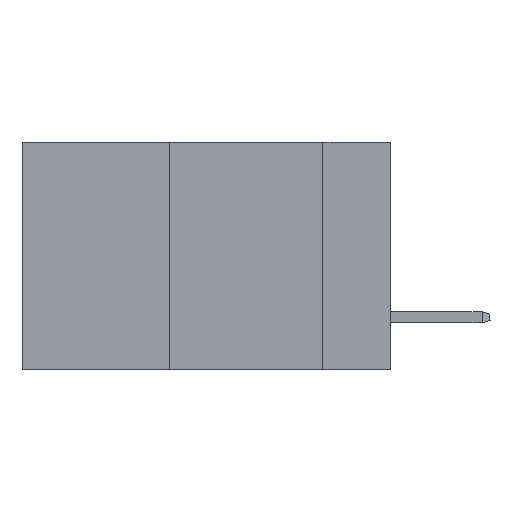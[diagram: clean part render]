
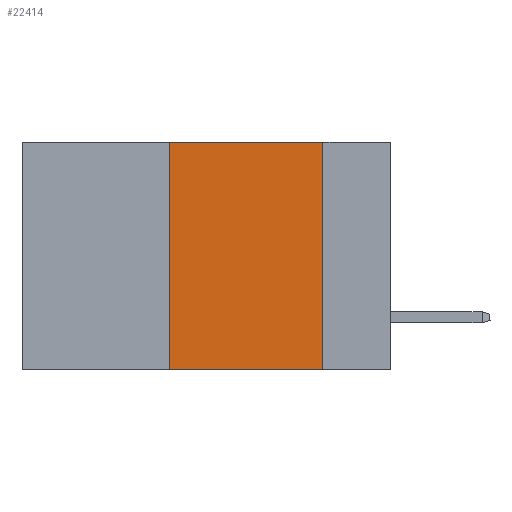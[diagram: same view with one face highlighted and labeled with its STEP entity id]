
A CAD part, left-side view. The second image highlights one B-rep face of the part: STEP entity #22414.
In plain terms, the highlighted planar face has unit normal (-1, 0, 0).
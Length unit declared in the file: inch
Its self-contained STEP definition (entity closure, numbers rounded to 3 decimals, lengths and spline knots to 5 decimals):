
#625 = DIRECTION ( 'NONE',  ( 0., 0., 1. ) ) ;
#879 = LINE ( 'NONE', #35204, #22034 ) ;
#1577 = VECTOR ( 'NONE', #19397, 39.37008 ) ;
#3331 = DIRECTION ( 'NONE',  ( 0., -1., 0. ) ) ;
#5216 = VECTOR ( 'NONE', #625, 39.37008 ) ;
#8493 = CARTESIAN_POINT ( 'NONE',  ( 0., 0.6, 0. ) ) ;
#9278 = CARTESIAN_POINT ( 'NONE',  ( 0., 0.36, 0. ) ) ;
#14355 = VECTOR ( 'NONE', #3331, 39.37008 ) ;
#16686 = AXIS2_PLACEMENT_3D ( 'NONE', #8493, #32992, #22421 ) ;
#19397 = DIRECTION ( 'NONE',  ( 0., 0., -1. ) ) ;
#21113 = LINE ( 'NONE', #22039, #1577 ) ;
#22034 = VECTOR ( 'NONE', #28789, 39.37008 ) ;
#22039 = CARTESIAN_POINT ( 'NONE',  ( 0., 0.11, 0. ) ) ;
#22054 = CARTESIAN_POINT ( 'NONE',  ( 0., 0.11, 0. ) ) ;
#22414 = ADVANCED_FACE ( 'NONE', ( #29050 ), #33474, .F. ) ;
#22421 = DIRECTION ( 'NONE',  ( 0., 0., -1. ) ) ;
#23936 = EDGE_CURVE ( 'NONE', #31148, #43775, #21113, .T. ) ;
#25295 = ORIENTED_EDGE ( 'NONE', *, *, #36280, .T. ) ;
#25302 = VERTEX_POINT ( 'NONE', #30016 ) ;
#25408 = LINE ( 'NONE', #45406, #14355 ) ;
#27112 = EDGE_LOOP ( 'NONE', ( #36777, #28800, #43713, #25295 ) ) ;
#28789 = DIRECTION ( 'NONE',  ( 0., -1., 0. ) ) ;
#28800 = ORIENTED_EDGE ( 'NONE', *, *, #32764, .F. ) ;
#29050 = FACE_OUTER_BOUND ( 'NONE', #27112, .T. ) ;
#29289 = EDGE_CURVE ( 'NONE', #25302, #40293, #31388, .T. ) ;
#30016 = CARTESIAN_POINT ( 'NONE',  ( 0., 0.36, -0.37 ) ) ;
#31148 = VERTEX_POINT ( 'NONE', #22054 ) ;
#31388 = LINE ( 'NONE', #36402, #5216 ) ;
#32764 = EDGE_CURVE ( 'NONE', #40293, #31148, #25408, .T. ) ;
#32992 = DIRECTION ( 'NONE',  ( 1., 0., 0. ) ) ;
#33474 = PLANE ( 'NONE',  #16686 ) ;
#35204 = CARTESIAN_POINT ( 'NONE',  ( 0., 0.6, -0.37 ) ) ;
#36280 = EDGE_CURVE ( 'NONE', #25302, #43775, #879, .T. ) ;
#36402 = CARTESIAN_POINT ( 'NONE',  ( 0., 0.36, 0. ) ) ;
#36777 = ORIENTED_EDGE ( 'NONE', *, *, #23936, .F. ) ;
#39358 = CARTESIAN_POINT ( 'NONE',  ( 0., 0.11, -0.37 ) ) ;
#40293 = VERTEX_POINT ( 'NONE', #9278 ) ;
#43713 = ORIENTED_EDGE ( 'NONE', *, *, #29289, .F. ) ;
#43775 = VERTEX_POINT ( 'NONE', #39358 ) ;
#45406 = CARTESIAN_POINT ( 'NONE',  ( 0., 0.6, 0. ) ) ;
